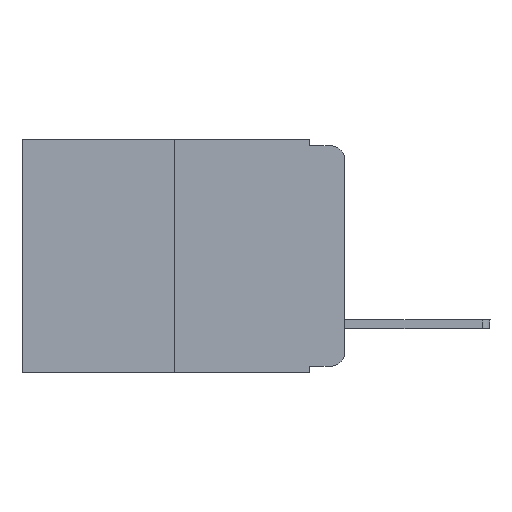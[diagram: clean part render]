
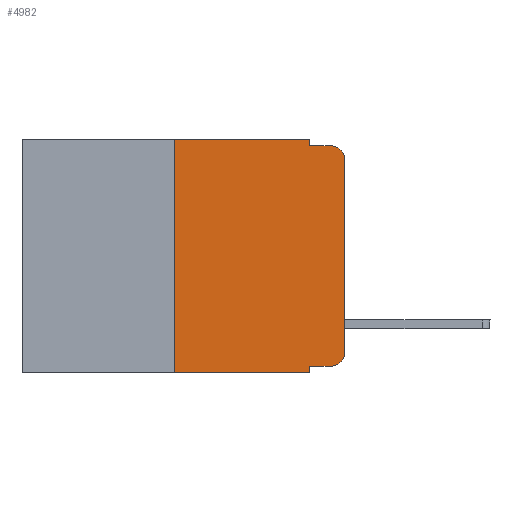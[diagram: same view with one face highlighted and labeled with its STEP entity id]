
A CAD part, left-side view. The second image highlights one B-rep face of the part: STEP entity #4982.
In plain terms, the highlighted planar face has unit normal (-1, 0, 0).
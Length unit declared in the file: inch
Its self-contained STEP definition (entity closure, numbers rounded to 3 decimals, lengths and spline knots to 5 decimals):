
#76 = ORIENTED_EDGE ( 'NONE', *, *, #17733, .F. ) ;
#348 = EDGE_CURVE ( 'NONE', #20531, #18135, #4973, .T. ) ;
#502 = CARTESIAN_POINT ( 'NONE',  ( 0., 0.25, -0.343 ) ) ;
#523 = EDGE_LOOP ( 'NONE', ( #12393, #22115, #24680, #8491, #76, #3076, #16445, #5771, #18226, #15241 ) ) ;
#757 = LINE ( 'NONE', #7857, #22616 ) ;
#940 = EDGE_CURVE ( 'NONE', #7273, #11173, #1242, .T. ) ;
#952 = DIRECTION ( 'NONE',  ( 0., -1., 0. ) ) ;
#1069 = VERTEX_POINT ( 'NONE', #15510 ) ;
#1158 = CARTESIAN_POINT ( 'NONE',  ( 0., 0., -0.03 ) ) ;
#1242 = CIRCLE ( 'NONE', #24046, 0.02 ) ;
#1250 = VERTEX_POINT ( 'NONE', #18684 ) ;
#1296 = CARTESIAN_POINT ( 'NONE',  ( 0., 0., 0. ) ) ;
#1410 = DIRECTION ( 'NONE',  ( 0., 0., 1. ) ) ;
#1413 = AXIS2_PLACEMENT_3D ( 'NONE', #15183, #15092, #3434 ) ;
#1674 = EDGE_CURVE ( 'NONE', #23276, #19511, #11495, .T. ) ;
#1783 = DIRECTION ( 'NONE',  ( 0., -1., 0. ) ) ;
#2027 = FACE_OUTER_BOUND ( 'NONE', #523, .T. ) ;
#2384 = DIRECTION ( 'NONE',  ( 0., -1., 0. ) ) ;
#2658 = CARTESIAN_POINT ( 'NONE',  ( 0., 0.051, 0. ) ) ;
#2835 = EDGE_CURVE ( 'NONE', #1069, #11691, #23568, .T. ) ;
#3019 = DIRECTION ( 'NONE',  ( 0., 0., 1. ) ) ;
#3076 = ORIENTED_EDGE ( 'NONE', *, *, #10671, .F. ) ;
#3256 = VECTOR ( 'NONE', #2384, 39.37008 ) ;
#3434 = DIRECTION ( 'NONE',  ( 0., 0., -1. ) ) ;
#3895 = LINE ( 'NONE', #23795, #3256 ) ;
#4226 = VECTOR ( 'NONE', #16494, 39.37008 ) ;
#4524 = LINE ( 'NONE', #12965, #23593 ) ;
#4973 = LINE ( 'NONE', #8083, #24327 ) ;
#4982 = ADVANCED_FACE ( 'NONE', ( #2027 ), #5570, .F. ) ;
#5203 = EDGE_CURVE ( 'NONE', #18135, #11173, #3895, .T. ) ;
#5570 = PLANE ( 'NONE',  #1413 ) ;
#5771 = ORIENTED_EDGE ( 'NONE', *, *, #24096, .F. ) ;
#6074 = DIRECTION ( 'NONE',  ( 0., -1., 0. ) ) ;
#6954 = LINE ( 'NONE', #24429, #4226 ) ;
#7273 = VERTEX_POINT ( 'NONE', #1158 ) ;
#7857 = CARTESIAN_POINT ( 'NONE',  ( 0., 0.473, 0. ) ) ;
#7880 = CARTESIAN_POINT ( 'NONE',  ( 0., 0.051, -0.333 ) ) ;
#8083 = CARTESIAN_POINT ( 'NONE',  ( 0., 0.051, 0. ) ) ;
#8491 = ORIENTED_EDGE ( 'NONE', *, *, #348, .F. ) ;
#8588 = EDGE_CURVE ( 'NONE', #11691, #7273, #25187, .T. ) ;
#9178 = VECTOR ( 'NONE', #3019, 39.37008 ) ;
#9559 = CARTESIAN_POINT ( 'NONE',  ( 0., 0.051, -0.343 ) ) ;
#9680 = VERTEX_POINT ( 'NONE', #17900 ) ;
#10671 = EDGE_CURVE ( 'NONE', #23276, #1250, #4524, .T. ) ;
#10880 = VECTOR ( 'NONE', #952, 39.37008 ) ;
#11162 = CARTESIAN_POINT ( 'NONE',  ( 0., 0.051, -0.01 ) ) ;
#11173 = VERTEX_POINT ( 'NONE', #11564 ) ;
#11248 = DIRECTION ( 'NONE',  ( 0., 0., -1. ) ) ;
#11298 = DIRECTION ( 'NONE',  ( 0., 0., -1. ) ) ;
#11328 = DIRECTION ( 'NONE',  ( -1., 0., 0. ) ) ;
#11495 = LINE ( 'NONE', #18823, #10880 ) ;
#11564 = CARTESIAN_POINT ( 'NONE',  ( 0., 0.02, -0.01 ) ) ;
#11691 = VERTEX_POINT ( 'NONE', #22896 ) ;
#12393 = ORIENTED_EDGE ( 'NONE', *, *, #8588, .T. ) ;
#12965 = CARTESIAN_POINT ( 'NONE',  ( 0., 0.25, 0. ) ) ;
#13910 = EDGE_CURVE ( 'NONE', #9680, #1069, #21219, .T. ) ;
#15092 = DIRECTION ( 'NONE',  ( 1., 0., 0. ) ) ;
#15183 = CARTESIAN_POINT ( 'NONE',  ( 0., 0.473, 0. ) ) ;
#15241 = ORIENTED_EDGE ( 'NONE', *, *, #2835, .T. ) ;
#15510 = CARTESIAN_POINT ( 'NONE',  ( 0., 0.02, -0.333 ) ) ;
#16445 = ORIENTED_EDGE ( 'NONE', *, *, #1674, .T. ) ;
#16494 = DIRECTION ( 'NONE',  ( 0., 0., -1. ) ) ;
#17108 = CARTESIAN_POINT ( 'NONE',  ( 0., 0.02, -0.313 ) ) ;
#17653 = AXIS2_PLACEMENT_3D ( 'NONE', #17108, #11328, #11248 ) ;
#17733 = EDGE_CURVE ( 'NONE', #1250, #20531, #757, .T. ) ;
#17900 = CARTESIAN_POINT ( 'NONE',  ( 0., 0.051, -0.333 ) ) ;
#18078 = DIRECTION ( 'NONE',  ( 0., 0., -1. ) ) ;
#18135 = VERTEX_POINT ( 'NONE', #11162 ) ;
#18226 = ORIENTED_EDGE ( 'NONE', *, *, #13910, .T. ) ;
#18684 = CARTESIAN_POINT ( 'NONE',  ( 0., 0.25, 0. ) ) ;
#18823 = CARTESIAN_POINT ( 'NONE',  ( 0., 0.473, -0.343 ) ) ;
#19511 = VERTEX_POINT ( 'NONE', #9559 ) ;
#20531 = VERTEX_POINT ( 'NONE', #2658 ) ;
#21219 = LINE ( 'NONE', #7880, #21535 ) ;
#21228 = CARTESIAN_POINT ( 'NONE',  ( 0., 0.02, -0.03 ) ) ;
#21535 = VECTOR ( 'NONE', #6074, 39.37008 ) ;
#22115 = ORIENTED_EDGE ( 'NONE', *, *, #940, .T. ) ;
#22616 = VECTOR ( 'NONE', #1783, 39.37008 ) ;
#22896 = CARTESIAN_POINT ( 'NONE',  ( 0., 0., -0.313 ) ) ;
#23026 = DIRECTION ( 'NONE',  ( -1., 0., 0. ) ) ;
#23276 = VERTEX_POINT ( 'NONE', #502 ) ;
#23568 = CIRCLE ( 'NONE', #17653, 0.02 ) ;
#23593 = VECTOR ( 'NONE', #1410, 39.37008 ) ;
#23795 = CARTESIAN_POINT ( 'NONE',  ( 0., 0.051, -0.01 ) ) ;
#24046 = AXIS2_PLACEMENT_3D ( 'NONE', #21228, #23026, #11298 ) ;
#24096 = EDGE_CURVE ( 'NONE', #9680, #19511, #6954, .T. ) ;
#24327 = VECTOR ( 'NONE', #18078, 39.37008 ) ;
#24429 = CARTESIAN_POINT ( 'NONE',  ( 0., 0.051, 0. ) ) ;
#24680 = ORIENTED_EDGE ( 'NONE', *, *, #5203, .F. ) ;
#25187 = LINE ( 'NONE', #1296, #9178 ) ;
